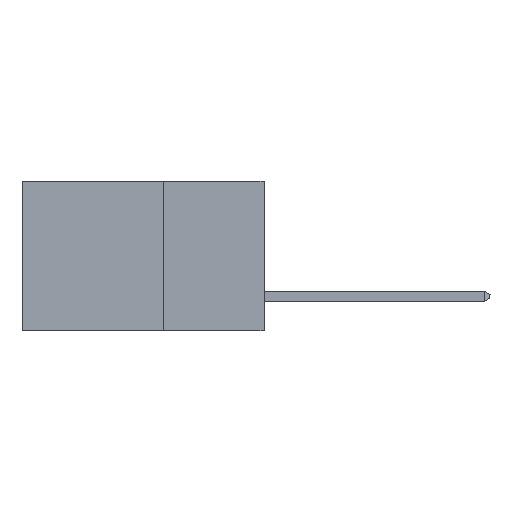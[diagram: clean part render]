
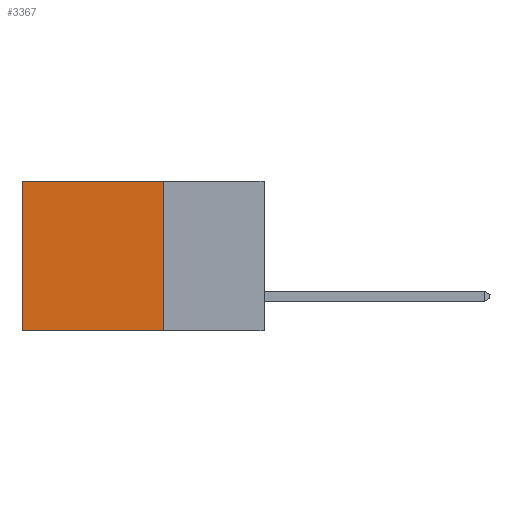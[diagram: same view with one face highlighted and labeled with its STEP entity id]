
A CAD part, left-side view. The second image highlights one B-rep face of the part: STEP entity #3367.
In plain terms, the highlighted planar face has unit normal (-1, 0, 0).
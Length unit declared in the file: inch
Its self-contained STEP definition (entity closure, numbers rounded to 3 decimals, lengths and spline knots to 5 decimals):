
#105 = CARTESIAN_POINT ( 'NONE',  ( 0.2615, 0.6, -0.37 ) ) ;
#242 = VECTOR ( 'NONE', #11781, 39.37008 ) ;
#588 = CARTESIAN_POINT ( 'NONE',  ( 0.2615, 0.6, 0. ) ) ;
#598 = ORIENTED_EDGE ( 'NONE', *, *, #8172, .T. ) ;
#1134 = VECTOR ( 'NONE', #13207, 39.37008 ) ;
#1680 = ORIENTED_EDGE ( 'NONE', *, *, #7890, .F. ) ;
#1704 = VERTEX_POINT ( 'NONE', #588 ) ;
#1756 = VECTOR ( 'NONE', #12307, 39.37008 ) ;
#1871 = PLANE ( 'NONE',  #5163 ) ;
#2402 = VERTEX_POINT ( 'NONE', #2673 ) ;
#2426 = CARTESIAN_POINT ( 'NONE',  ( 0.2615, 0.25, -0.37 ) ) ;
#2474 = EDGE_LOOP ( 'NONE', ( #9411, #4910, #1680, #598 ) ) ;
#2673 = CARTESIAN_POINT ( 'NONE',  ( 0.2615, 0.25, -0.37 ) ) ;
#2709 = EDGE_CURVE ( 'NONE', #1704, #11750, #9718, .T. ) ;
#2894 = LINE ( 'NONE', #7178, #13457 ) ;
#2995 = EDGE_CURVE ( 'NONE', #2402, #11750, #6860, .T. ) ;
#3367 = ADVANCED_FACE ( 'NONE', ( #4640 ), #1871, .F. ) ;
#4147 = DIRECTION ( 'NONE',  ( 0., 0., -1. ) ) ;
#4180 = CARTESIAN_POINT ( 'NONE',  ( 0.2615, 0.25, -0.37 ) ) ;
#4640 = FACE_OUTER_BOUND ( 'NONE', #2474, .T. ) ;
#4910 = ORIENTED_EDGE ( 'NONE', *, *, #2995, .F. ) ;
#5163 = AXIS2_PLACEMENT_3D ( 'NONE', #4180, #8278, #12584 ) ;
#6860 = LINE ( 'NONE', #2426, #1134 ) ;
#7178 = CARTESIAN_POINT ( 'NONE',  ( 0.2615, 0.25, -0.37 ) ) ;
#7890 = EDGE_CURVE ( 'NONE', #8932, #2402, #2894, .T. ) ;
#8140 = LINE ( 'NONE', #10454, #1756 ) ;
#8172 = EDGE_CURVE ( 'NONE', #8932, #1704, #8140, .T. ) ;
#8278 = DIRECTION ( 'NONE',  ( 1., 0., 0. ) ) ;
#8932 = VERTEX_POINT ( 'NONE', #11720 ) ;
#9411 = ORIENTED_EDGE ( 'NONE', *, *, #2709, .T. ) ;
#9718 = LINE ( 'NONE', #105, #242 ) ;
#10454 = CARTESIAN_POINT ( 'NONE',  ( 0.2615, 0.25, 0. ) ) ;
#11720 = CARTESIAN_POINT ( 'NONE',  ( 0.2615, 0.25, 0. ) ) ;
#11750 = VERTEX_POINT ( 'NONE', #13238 ) ;
#11781 = DIRECTION ( 'NONE',  ( 0., 0., -1. ) ) ;
#12307 = DIRECTION ( 'NONE',  ( 0., 1., 0. ) ) ;
#12584 = DIRECTION ( 'NONE',  ( 0., 0., -1. ) ) ;
#13207 = DIRECTION ( 'NONE',  ( 0., 1., 0. ) ) ;
#13238 = CARTESIAN_POINT ( 'NONE',  ( 0.2615, 0.6, -0.37 ) ) ;
#13457 = VECTOR ( 'NONE', #4147, 39.37008 ) ;
